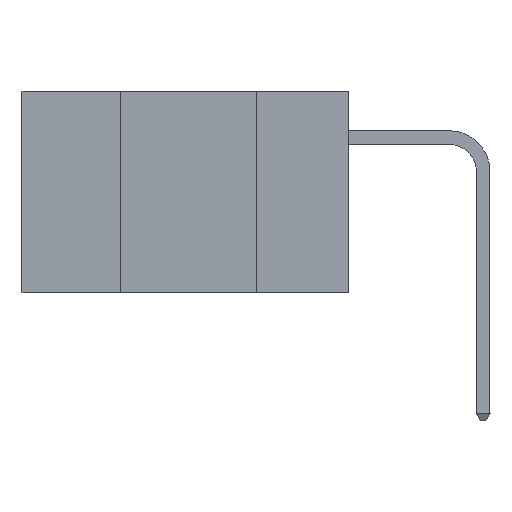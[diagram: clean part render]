
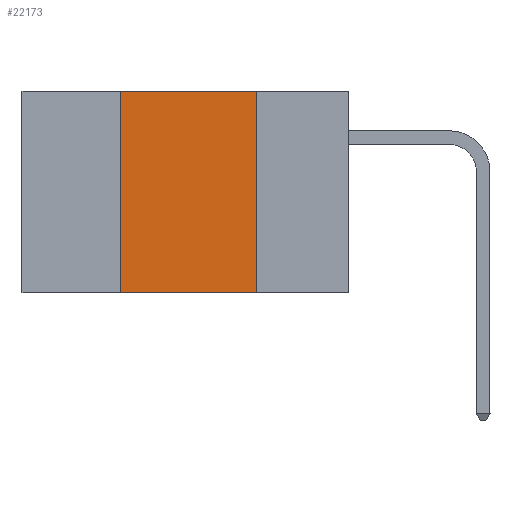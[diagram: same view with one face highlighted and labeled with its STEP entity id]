
A CAD part, left-side view. The second image highlights one B-rep face of the part: STEP entity #22173.
In plain terms, the highlighted planar face has unit normal (-1, 0, 0).
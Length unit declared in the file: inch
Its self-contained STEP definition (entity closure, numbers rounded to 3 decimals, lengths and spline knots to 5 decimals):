
#236 = CARTESIAN_POINT ( 'NONE',  ( 0., 0.17, -0.37 ) ) ;
#1475 = VERTEX_POINT ( 'NONE', #4849 ) ;
#1591 = CARTESIAN_POINT ( 'NONE',  ( 0., 0.17, 0. ) ) ;
#2164 = VERTEX_POINT ( 'NONE', #7830 ) ;
#2515 = ORIENTED_EDGE ( 'NONE', *, *, #21285, .T. ) ;
#4007 = VECTOR ( 'NONE', #18719, 39.37008 ) ;
#4849 = CARTESIAN_POINT ( 'NONE',  ( 0., 0.17, 0. ) ) ;
#5026 = VECTOR ( 'NONE', #13880, 39.37008 ) ;
#5072 = EDGE_CURVE ( 'NONE', #1475, #9595, #11633, .T. ) ;
#6552 = FACE_OUTER_BOUND ( 'NONE', #16249, .T. ) ;
#7830 = CARTESIAN_POINT ( 'NONE',  ( 0., 0.42, -0.37 ) ) ;
#7919 = VECTOR ( 'NONE', #19670, 39.37008 ) ;
#8917 = EDGE_CURVE ( 'NONE', #2164, #17532, #21872, .T. ) ;
#9389 = CARTESIAN_POINT ( 'NONE',  ( 0., 0.42, 0. ) ) ;
#9595 = VERTEX_POINT ( 'NONE', #236 ) ;
#11633 = LINE ( 'NONE', #1591, #7919 ) ;
#12489 = CARTESIAN_POINT ( 'NONE',  ( 0., 0.6, 0. ) ) ;
#12876 = AXIS2_PLACEMENT_3D ( 'NONE', #12489, #14845, #22613 ) ;
#13166 = LINE ( 'NONE', #24780, #4007 ) ;
#13446 = CARTESIAN_POINT ( 'NONE',  ( 0., 0.42, 0. ) ) ;
#13880 = DIRECTION ( 'NONE',  ( 0., -1., 0. ) ) ;
#14588 = PLANE ( 'NONE',  #12876 ) ;
#14845 = DIRECTION ( 'NONE',  ( 1., 0., 0. ) ) ;
#15565 = DIRECTION ( 'NONE',  ( 0., 0., 1. ) ) ;
#16249 = EDGE_LOOP ( 'NONE', ( #22347, #20244, #25968, #2515 ) ) ;
#17435 = LINE ( 'NONE', #25866, #5026 ) ;
#17531 = EDGE_CURVE ( 'NONE', #17532, #1475, #17435, .T. ) ;
#17532 = VERTEX_POINT ( 'NONE', #9389 ) ;
#18719 = DIRECTION ( 'NONE',  ( 0., -1., 0. ) ) ;
#19670 = DIRECTION ( 'NONE',  ( 0., 0., -1. ) ) ;
#20244 = ORIENTED_EDGE ( 'NONE', *, *, #17531, .F. ) ;
#21285 = EDGE_CURVE ( 'NONE', #2164, #9595, #13166, .T. ) ;
#21872 = LINE ( 'NONE', #13446, #24954 ) ;
#22173 = ADVANCED_FACE ( 'NONE', ( #6552 ), #14588, .F. ) ;
#22347 = ORIENTED_EDGE ( 'NONE', *, *, #5072, .F. ) ;
#22613 = DIRECTION ( 'NONE',  ( 0., 0., -1. ) ) ;
#24780 = CARTESIAN_POINT ( 'NONE',  ( 0., 0.6, -0.37 ) ) ;
#24954 = VECTOR ( 'NONE', #15565, 39.37008 ) ;
#25866 = CARTESIAN_POINT ( 'NONE',  ( 0., 0.6, 0. ) ) ;
#25968 = ORIENTED_EDGE ( 'NONE', *, *, #8917, .F. ) ;
